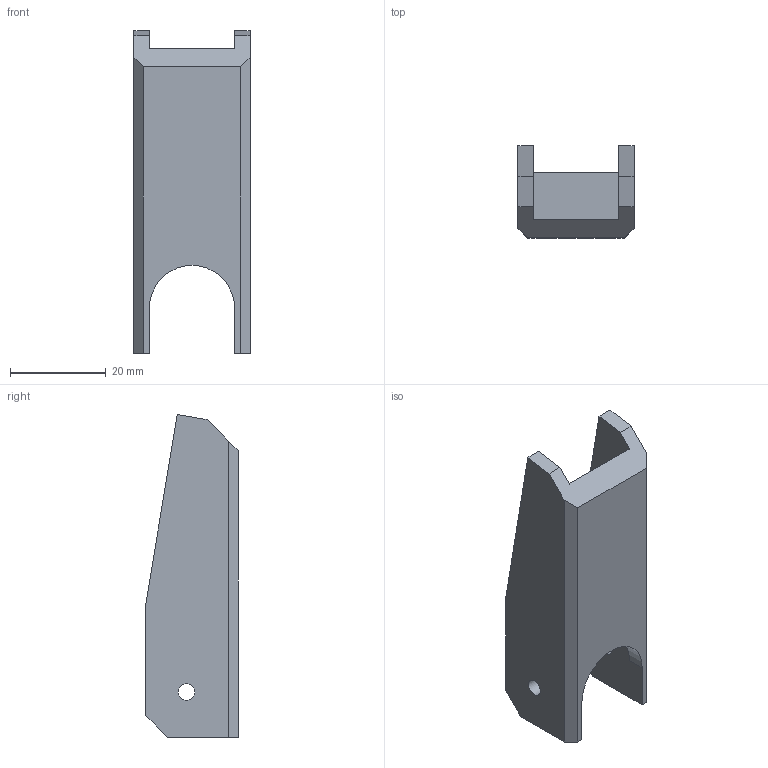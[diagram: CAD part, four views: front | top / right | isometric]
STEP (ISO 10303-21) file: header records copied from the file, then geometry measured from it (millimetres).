
FILE_DESCRIPTION( ( '' ), ' ' );
FILE_NAME( '5dc6e51b9433371275628cce.step', '2019-11-09T16:11:08', ( '' ), ( '' ), ' ', ' ', ' ' );
FILE_SCHEMA( ( 'AUTOMOTIVE_DESIGN { 1 0 10303 214 1 1 1 1 }' ) );
Length unit declared in the file: metre
Products named in the file (1): Part 1
Bounding box: 24.3 x 19.3 x 67.5 mm (x, y, z)
Volume: 10740.8 mm3; surface area: 7152.9 mm2
Topology: 1 solids, 1 shells, 26 faces, 74 edges, 50 vertices
Faces by surface type: plane 23, cylinder 3
Full cylindrical faces by diameter (mm): 3.5 x2
Entity records: 1044 total; most frequent: CARTESIAN_POINT 145, ORIENTED_EDGE 140, DIRECTION 130, EDGE_CURVE 70, LINE 64, VECTOR 64, VERTEX_POINT 48, AXIS2_PLACEMENT_3D 33
